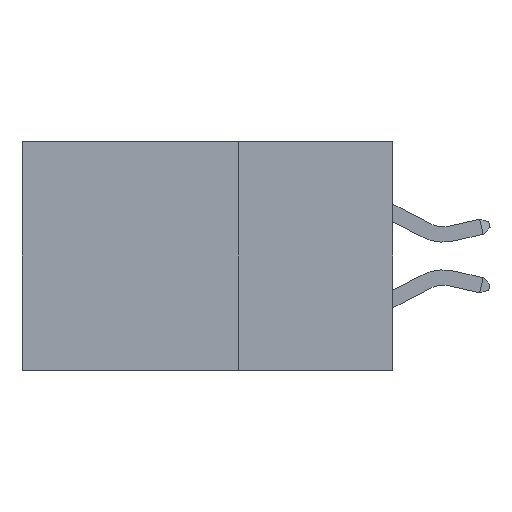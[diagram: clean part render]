
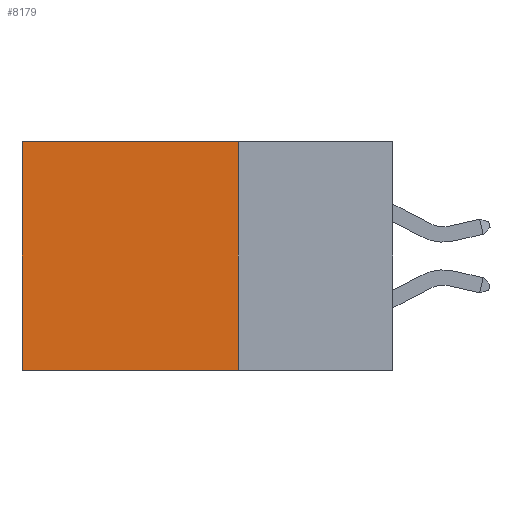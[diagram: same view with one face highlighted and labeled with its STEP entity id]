
A CAD part, left-side view. The second image highlights one B-rep face of the part: STEP entity #8179.
In plain terms, the highlighted planar face has unit normal (-1, 0, 0).
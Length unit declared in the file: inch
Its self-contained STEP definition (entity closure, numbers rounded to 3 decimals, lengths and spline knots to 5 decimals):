
#162 = LINE ( 'NONE', #8572, #3564 ) ;
#351 = VECTOR ( 'NONE', #5164, 39.37008 ) ;
#868 = EDGE_CURVE ( 'NONE', #17068, #13643, #162, .T. ) ;
#1111 = DIRECTION ( 'NONE',  ( 1., 0., 0. ) ) ;
#1277 = CARTESIAN_POINT ( 'NONE',  ( 0.2875, 0.6, -0.37 ) ) ;
#1627 = DIRECTION ( 'NONE',  ( 0., 1., 0. ) ) ;
#1918 = VERTEX_POINT ( 'NONE', #9199 ) ;
#3357 = VECTOR ( 'NONE', #11334, 39.37008 ) ;
#3564 = VECTOR ( 'NONE', #1627, 39.37008 ) ;
#4499 = AXIS2_PLACEMENT_3D ( 'NONE', #7947, #1111, #16524 ) ;
#5164 = DIRECTION ( 'NONE',  ( 0., 0., -1. ) ) ;
#5376 = VERTEX_POINT ( 'NONE', #8439 ) ;
#5389 = EDGE_CURVE ( 'NONE', #1918, #13643, #17440, .T. ) ;
#5561 = CARTESIAN_POINT ( 'NONE',  ( 0.2875, 0.25, 0. ) ) ;
#6061 = EDGE_CURVE ( 'NONE', #5376, #17068, #13566, .T. ) ;
#6553 = VECTOR ( 'NONE', #17169, 39.37008 ) ;
#7115 = LINE ( 'NONE', #5561, #3357 ) ;
#7502 = CARTESIAN_POINT ( 'NONE',  ( 0.2875, 0.6, 0. ) ) ;
#7947 = CARTESIAN_POINT ( 'NONE',  ( 0.2875, 0.25, 0. ) ) ;
#8179 = ADVANCED_FACE ( 'NONE', ( #17786 ), #12148, .F. ) ;
#8253 = CARTESIAN_POINT ( 'NONE',  ( 0.2875, 0.25, -0.37 ) ) ;
#8439 = CARTESIAN_POINT ( 'NONE',  ( 0.2875, 0.25, 0. ) ) ;
#8572 = CARTESIAN_POINT ( 'NONE',  ( 0.2875, 0.25, -0.37 ) ) ;
#9199 = CARTESIAN_POINT ( 'NONE',  ( 0.2875, 0.6, 0. ) ) ;
#9871 = ORIENTED_EDGE ( 'NONE', *, *, #10781, .T. ) ;
#10781 = EDGE_CURVE ( 'NONE', #5376, #1918, #7115, .T. ) ;
#11334 = DIRECTION ( 'NONE',  ( 0., 1., 0. ) ) ;
#12148 = PLANE ( 'NONE',  #4499 ) ;
#12220 = ORIENTED_EDGE ( 'NONE', *, *, #6061, .F. ) ;
#13019 = EDGE_LOOP ( 'NONE', ( #15311, #13262, #12220, #9871 ) ) ;
#13262 = ORIENTED_EDGE ( 'NONE', *, *, #868, .F. ) ;
#13566 = LINE ( 'NONE', #17652, #351 ) ;
#13643 = VERTEX_POINT ( 'NONE', #1277 ) ;
#15311 = ORIENTED_EDGE ( 'NONE', *, *, #5389, .T. ) ;
#16524 = DIRECTION ( 'NONE',  ( 0., 0., -1. ) ) ;
#17068 = VERTEX_POINT ( 'NONE', #8253 ) ;
#17169 = DIRECTION ( 'NONE',  ( 0., 0., -1. ) ) ;
#17440 = LINE ( 'NONE', #7502, #6553 ) ;
#17652 = CARTESIAN_POINT ( 'NONE',  ( 0.2875, 0.25, 0. ) ) ;
#17786 = FACE_OUTER_BOUND ( 'NONE', #13019, .T. ) ;
